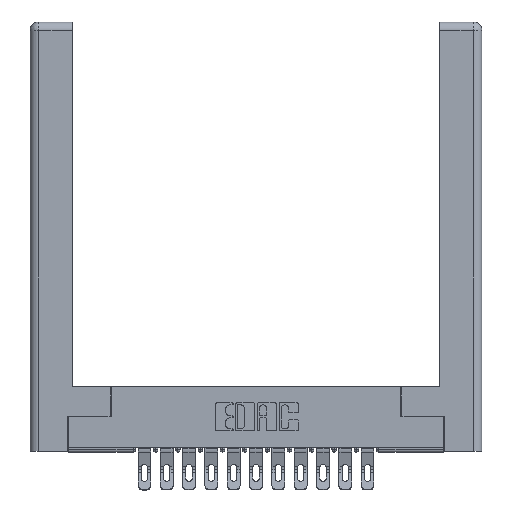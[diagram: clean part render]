
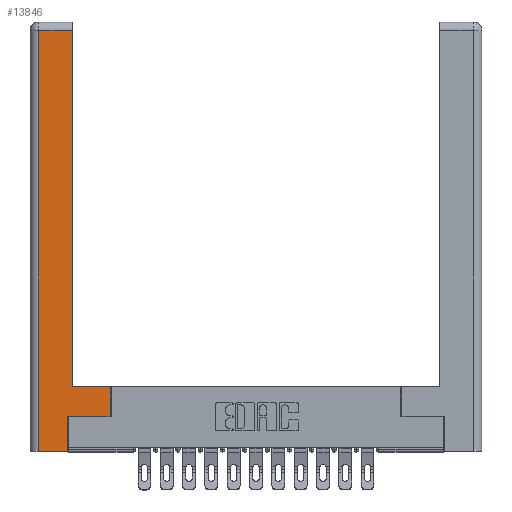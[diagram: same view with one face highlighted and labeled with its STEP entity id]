
A CAD part, top view. The second image highlights one B-rep face of the part: STEP entity #13846.
In plain terms, the highlighted planar face has unit normal (0, 0, 1).
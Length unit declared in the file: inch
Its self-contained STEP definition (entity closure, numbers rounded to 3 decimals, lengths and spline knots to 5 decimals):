
#13 = CARTESIAN_POINT ( 'NONE',  ( 0.265, 0.245, 0. ) ) ;
#29 = VECTOR ( 'NONE', #13251, 39.37008 ) ;
#127 = FACE_OUTER_BOUND ( 'NONE', #11611, .T. ) ;
#345 = VECTOR ( 'NONE', #8975, 39.37008 ) ;
#687 = DIRECTION ( 'NONE',  ( -1., 0., 0. ) ) ;
#1196 = VECTOR ( 'NONE', #15499, 39.37008 ) ;
#1369 = CARTESIAN_POINT ( 'NONE',  ( 0.565, 0.245, 0. ) ) ;
#1499 = VECTOR ( 'NONE', #11750, 39.37008 ) ;
#2241 = VECTOR ( 'NONE', #17595, 39.37008 ) ;
#2257 = EDGE_CURVE ( 'NONE', #4950, #18032, #2348, .T. ) ;
#2348 = LINE ( 'NONE', #2636, #17481 ) ;
#2636 = CARTESIAN_POINT ( 'NONE',  ( 0.265, 0.245, 0. ) ) ;
#2987 = CARTESIAN_POINT ( 'NONE',  ( 0.295, 3., 0. ) ) ;
#3170 = VERTEX_POINT ( 'NONE', #5258 ) ;
#3457 = EDGE_CURVE ( 'NONE', #16570, #4372, #16993, .T. ) ;
#4215 = CARTESIAN_POINT ( 'NONE',  ( 0.295, 0.45, 0. ) ) ;
#4372 = VERTEX_POINT ( 'NONE', #14438 ) ;
#4387 = VECTOR ( 'NONE', #7535, 39.37008 ) ;
#4499 = CARTESIAN_POINT ( 'NONE',  ( 0.565, 0.45, 0. ) ) ;
#4593 = CARTESIAN_POINT ( 'NONE',  ( 0.265, 0., 0. ) ) ;
#4950 = VERTEX_POINT ( 'NONE', #11865 ) ;
#5065 = CARTESIAN_POINT ( 'NONE',  ( 0.0615, 2.94, 0. ) ) ;
#5258 = CARTESIAN_POINT ( 'NONE',  ( 0.295, 2.94, 0. ) ) ;
#5465 = LINE ( 'NONE', #11658, #2241 ) ;
#5582 = VERTEX_POINT ( 'NONE', #5065 ) ;
#5778 = LINE ( 'NONE', #17102, #1196 ) ;
#7474 = VECTOR ( 'NONE', #10222, 39.37008 ) ;
#7535 = DIRECTION ( 'NONE',  ( 0., 1., 0. ) ) ;
#8204 = EDGE_CURVE ( 'NONE', #5582, #17074, #8385, .T. ) ;
#8385 = LINE ( 'NONE', #12841, #1499 ) ;
#8874 = EDGE_CURVE ( 'NONE', #17074, #4950, #13867, .T. ) ;
#8888 = ORIENTED_EDGE ( 'NONE', *, *, #8204, .T. ) ;
#8975 = DIRECTION ( 'NONE',  ( 1., 0., 0. ) ) ;
#9127 = ORIENTED_EDGE ( 'NONE', *, *, #9642, .T. ) ;
#9472 = DIRECTION ( 'NONE',  ( 0., 0., -1. ) ) ;
#9491 = DIRECTION ( 'NONE',  ( 0., 1., 0. ) ) ;
#9642 = EDGE_CURVE ( 'NONE', #18032, #16570, #17524, .T. ) ;
#9714 = ORIENTED_EDGE ( 'NONE', *, *, #8874, .T. ) ;
#10222 = DIRECTION ( 'NONE',  ( 1., 0., 0. ) ) ;
#10758 = CARTESIAN_POINT ( 'NONE',  ( 0., 0., 0. ) ) ;
#10887 = AXIS2_PLACEMENT_3D ( 'NONE', #10758, #9472, #687 ) ;
#11203 = ORIENTED_EDGE ( 'NONE', *, *, #16458, .T. ) ;
#11360 = CARTESIAN_POINT ( 'NONE',  ( 0.0615, 0., 0. ) ) ;
#11584 = ORIENTED_EDGE ( 'NONE', *, *, #3457, .T. ) ;
#11611 = EDGE_LOOP ( 'NONE', ( #11203, #14391, #8888, #9714, #16881, #9127, #11584, #12370 ) ) ;
#11658 = CARTESIAN_POINT ( 'NONE',  ( 0.295, 0.45, 0. ) ) ;
#11750 = DIRECTION ( 'NONE',  ( 0., -1., 0. ) ) ;
#11865 = CARTESIAN_POINT ( 'NONE',  ( 0.265, 0., 0. ) ) ;
#12140 = CARTESIAN_POINT ( 'NONE',  ( 0.565, 0.245, 0. ) ) ;
#12228 = PLANE ( 'NONE',  #10887 ) ;
#12370 = ORIENTED_EDGE ( 'NONE', *, *, #18003, .T. ) ;
#12841 = CARTESIAN_POINT ( 'NONE',  ( 0.0615, 0., 0. ) ) ;
#13251 = DIRECTION ( 'NONE',  ( 0., 1., 0. ) ) ;
#13846 = ADVANCED_FACE ( 'NONE', ( #127 ), #12228, .F. ) ;
#13867 = LINE ( 'NONE', #4593, #345 ) ;
#14391 = ORIENTED_EDGE ( 'NONE', *, *, #15504, .T. ) ;
#14438 = CARTESIAN_POINT ( 'NONE',  ( 0.565, 0.45, 0. ) ) ;
#15499 = DIRECTION ( 'NONE',  ( -1., 0., 0. ) ) ;
#15504 = EDGE_CURVE ( 'NONE', #3170, #5582, #5778, .T. ) ;
#15859 = VERTEX_POINT ( 'NONE', #4215 ) ;
#16458 = EDGE_CURVE ( 'NONE', #15859, #3170, #17423, .T. ) ;
#16570 = VERTEX_POINT ( 'NONE', #12140 ) ;
#16881 = ORIENTED_EDGE ( 'NONE', *, *, #2257, .T. ) ;
#16993 = LINE ( 'NONE', #4499, #4387 ) ;
#17074 = VERTEX_POINT ( 'NONE', #11360 ) ;
#17102 = CARTESIAN_POINT ( 'NONE',  ( 0.0615, 2.94, 0. ) ) ;
#17423 = LINE ( 'NONE', #2987, #29 ) ;
#17481 = VECTOR ( 'NONE', #9491, 39.37008 ) ;
#17524 = LINE ( 'NONE', #1369, #7474 ) ;
#17595 = DIRECTION ( 'NONE',  ( -1., 0., 0. ) ) ;
#18003 = EDGE_CURVE ( 'NONE', #4372, #15859, #5465, .T. ) ;
#18032 = VERTEX_POINT ( 'NONE', #13 ) ;
